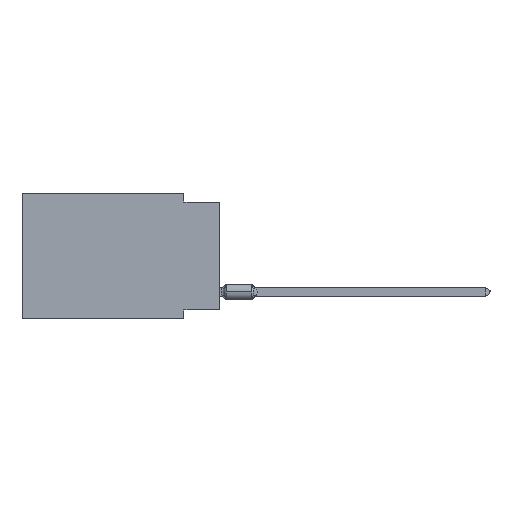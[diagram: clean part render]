
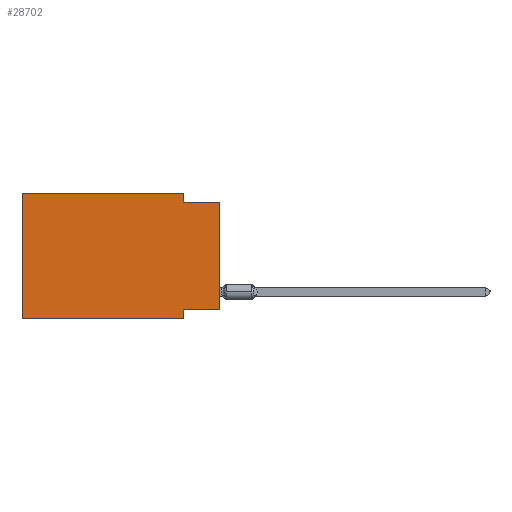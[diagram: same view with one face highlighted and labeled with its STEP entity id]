
A CAD part, left-side view. The second image highlights one B-rep face of the part: STEP entity #28702.
In plain terms, the highlighted planar face has unit normal (-1, 0, 0).
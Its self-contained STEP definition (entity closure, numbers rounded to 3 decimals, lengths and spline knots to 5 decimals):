
#543 = AXIS2_PLACEMENT_3D ( 'NONE', #23556, #10964, #24374 ) ;
#1525 = CARTESIAN_POINT ( 'NONE',  ( 0., 0., -0.025 ) ) ;
#2245 = VERTEX_POINT ( 'NONE', #11019 ) ;
#3187 = VERTEX_POINT ( 'NONE', #39303 ) ;
#3194 = CARTESIAN_POINT ( 'NONE',  ( 0., 0., 0. ) ) ;
#9083 = LINE ( 'NONE', #3194, #55980 ) ;
#10734 = VERTEX_POINT ( 'NONE', #23006 ) ;
#10842 = ORIENTED_EDGE ( 'NONE', *, *, #14576, .T. ) ;
#10964 = DIRECTION ( 'NONE',  ( 1., 0., 0. ) ) ;
#11019 = CARTESIAN_POINT ( 'NONE',  ( 0., 0., -0.025 ) ) ;
#11593 = CARTESIAN_POINT ( 'NONE',  ( 0., 0.1, -0.325 ) ) ;
#12029 = VERTEX_POINT ( 'NONE', #58778 ) ;
#12795 = VECTOR ( 'NONE', #70266, 39.37008 ) ;
#13170 = ORIENTED_EDGE ( 'NONE', *, *, #56050, .F. ) ;
#14576 = EDGE_CURVE ( 'NONE', #12029, #46979, #64364, .T. ) ;
#15320 = VECTOR ( 'NONE', #25841, 39.37008 ) ;
#16717 = ORIENTED_EDGE ( 'NONE', *, *, #58028, .F. ) ;
#19339 = DIRECTION ( 'NONE',  ( 0., 1., 0. ) ) ;
#20006 = DIRECTION ( 'NONE',  ( 0., -1., 0. ) ) ;
#21755 = CARTESIAN_POINT ( 'NONE',  ( 0., 0., -0.325 ) ) ;
#23006 = CARTESIAN_POINT ( 'NONE',  ( 0., 0.55, 0. ) ) ;
#23556 = CARTESIAN_POINT ( 'NONE',  ( 0., 0.55, 0. ) ) ;
#24145 = DIRECTION ( 'NONE',  ( 0., 0., -1. ) ) ;
#24374 = DIRECTION ( 'NONE',  ( 0., 0., -1. ) ) ;
#25108 = VECTOR ( 'NONE', #20006, 39.37008 ) ;
#25841 = DIRECTION ( 'NONE',  ( 0., -1., 0. ) ) ;
#28702 = ADVANCED_FACE ( 'NONE', ( #43681 ), #56241, .F. ) ;
#29597 = CARTESIAN_POINT ( 'NONE',  ( 0., 0.1, 0. ) ) ;
#30007 = ORIENTED_EDGE ( 'NONE', *, *, #68779, .F. ) ;
#33229 = EDGE_CURVE ( 'NONE', #46640, #3187, #61887, .T. ) ;
#33257 = DIRECTION ( 'NONE',  ( 0., 0., 1. ) ) ;
#35136 = EDGE_CURVE ( 'NONE', #3187, #2245, #77055, .T. ) ;
#36176 = DIRECTION ( 'NONE',  ( 0., 0., -1. ) ) ;
#36547 = EDGE_CURVE ( 'NONE', #64676, #2245, #9083, .T. ) ;
#39303 = CARTESIAN_POINT ( 'NONE',  ( 0., 0.1, -0.025 ) ) ;
#42060 = CARTESIAN_POINT ( 'NONE',  ( 0., 0.1, -0.35 ) ) ;
#43681 = FACE_OUTER_BOUND ( 'NONE', #71731, .T. ) ;
#43976 = ORIENTED_EDGE ( 'NONE', *, *, #72464, .F. ) ;
#46639 = ORIENTED_EDGE ( 'NONE', *, *, #36547, .T. ) ;
#46640 = VERTEX_POINT ( 'NONE', #74207 ) ;
#46753 = CARTESIAN_POINT ( 'NONE',  ( 0., 0.1, -0.35 ) ) ;
#46979 = VERTEX_POINT ( 'NONE', #46753 ) ;
#49891 = VECTOR ( 'NONE', #33257, 39.37008 ) ;
#52131 = LINE ( 'NONE', #77725, #49891 ) ;
#55058 = LINE ( 'NONE', #42060, #72273 ) ;
#55980 = VECTOR ( 'NONE', #61494, 39.37008 ) ;
#56050 = EDGE_CURVE ( 'NONE', #74651, #46979, #55058, .T. ) ;
#56241 = PLANE ( 'NONE',  #543 ) ;
#57273 = CARTESIAN_POINT ( 'NONE',  ( 0., 0.55, -0.35 ) ) ;
#57923 = CARTESIAN_POINT ( 'NONE',  ( 0., 0., -0.325 ) ) ;
#58028 = EDGE_CURVE ( 'NONE', #64676, #74651, #70903, .T. ) ;
#58778 = CARTESIAN_POINT ( 'NONE',  ( 0., 0.55, -0.35 ) ) ;
#61494 = DIRECTION ( 'NONE',  ( 0., 0., 1. ) ) ;
#61887 = LINE ( 'NONE', #29597, #63653 ) ;
#63653 = VECTOR ( 'NONE', #24145, 39.37008 ) ;
#64364 = LINE ( 'NONE', #57273, #12795 ) ;
#64676 = VERTEX_POINT ( 'NONE', #21755 ) ;
#65804 = VECTOR ( 'NONE', #19339, 39.37008 ) ;
#66116 = ORIENTED_EDGE ( 'NONE', *, *, #33229, .F. ) ;
#68779 = EDGE_CURVE ( 'NONE', #10734, #46640, #81663, .T. ) ;
#70266 = DIRECTION ( 'NONE',  ( 0., -1., 0. ) ) ;
#70903 = LINE ( 'NONE', #57923, #65804 ) ;
#71731 = EDGE_LOOP ( 'NONE', ( #46639, #78233, #66116, #30007, #43976, #10842, #13170, #16717 ) ) ;
#72273 = VECTOR ( 'NONE', #36176, 39.37008 ) ;
#72464 = EDGE_CURVE ( 'NONE', #12029, #10734, #52131, .T. ) ;
#74207 = CARTESIAN_POINT ( 'NONE',  ( 0., 0.1, 0. ) ) ;
#74651 = VERTEX_POINT ( 'NONE', #11593 ) ;
#77055 = LINE ( 'NONE', #1525, #25108 ) ;
#77725 = CARTESIAN_POINT ( 'NONE',  ( 0., 0.55, 0. ) ) ;
#78233 = ORIENTED_EDGE ( 'NONE', *, *, #35136, .F. ) ;
#81663 = LINE ( 'NONE', #82079, #15320 ) ;
#82079 = CARTESIAN_POINT ( 'NONE',  ( 0., 0.55, 0. ) ) ;
